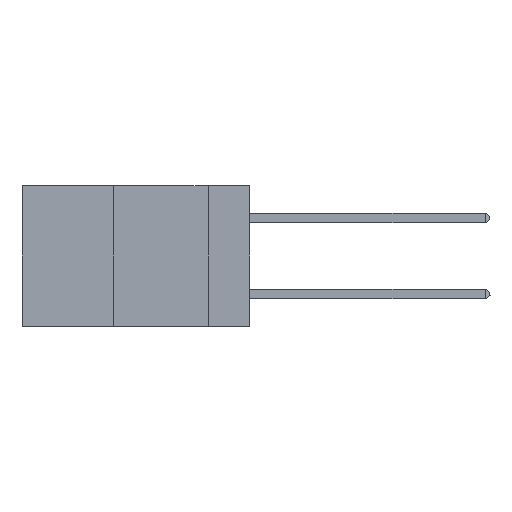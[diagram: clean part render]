
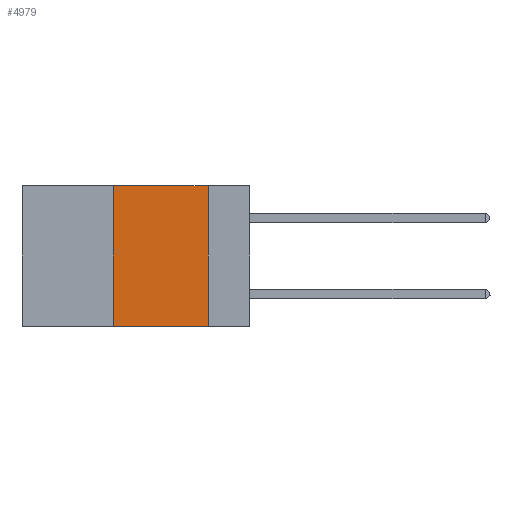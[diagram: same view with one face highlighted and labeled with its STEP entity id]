
A CAD part, left-side view. The second image highlights one B-rep face of the part: STEP entity #4979.
In plain terms, the highlighted planar face has unit normal (-1, 0, 0).
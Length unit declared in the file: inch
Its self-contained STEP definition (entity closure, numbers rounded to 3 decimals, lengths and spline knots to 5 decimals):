
#2656 = LINE ( 'NONE', #20775, #21269 ) ;
#2735 = VERTEX_POINT ( 'NONE', #14490 ) ;
#2810 = VECTOR ( 'NONE', #8553, 39.37008 ) ;
#2898 = CARTESIAN_POINT ( 'NONE',  ( 0., 0.36, 0. ) ) ;
#4979 = ADVANCED_FACE ( 'NONE', ( #11191 ), #26949, .F. ) ;
#6540 = VERTEX_POINT ( 'NONE', #43272 ) ;
#8553 = DIRECTION ( 'NONE',  ( 0., -1., 0. ) ) ;
#8748 = AXIS2_PLACEMENT_3D ( 'NONE', #21558, #14508, #42580 ) ;
#11191 = FACE_OUTER_BOUND ( 'NONE', #39008, .T. ) ;
#11654 = ORIENTED_EDGE ( 'NONE', *, *, #19521, .T. ) ;
#12310 = CARTESIAN_POINT ( 'NONE',  ( 0., 0.36, 0. ) ) ;
#14490 = CARTESIAN_POINT ( 'NONE',  ( 0., 0.36, -0.37 ) ) ;
#14508 = DIRECTION ( 'NONE',  ( 1., 0., 0. ) ) ;
#17548 = VECTOR ( 'NONE', #33337, 39.37008 ) ;
#18623 = VERTEX_POINT ( 'NONE', #24396 ) ;
#19521 = EDGE_CURVE ( 'NONE', #2735, #6540, #2656, .T. ) ;
#20775 = CARTESIAN_POINT ( 'NONE',  ( 0., 0.6, -0.37 ) ) ;
#21269 = VECTOR ( 'NONE', #37691, 39.37008 ) ;
#21558 = CARTESIAN_POINT ( 'NONE',  ( 0., 0.6, 0. ) ) ;
#21889 = VERTEX_POINT ( 'NONE', #12310 ) ;
#23025 = CARTESIAN_POINT ( 'NONE',  ( 0., 0.11, 0. ) ) ;
#23467 = VECTOR ( 'NONE', #35154, 39.37008 ) ;
#24396 = CARTESIAN_POINT ( 'NONE',  ( 0., 0.11, 0. ) ) ;
#25597 = ORIENTED_EDGE ( 'NONE', *, *, #35608, .F. ) ;
#26558 = ORIENTED_EDGE ( 'NONE', *, *, #31101, .F. ) ;
#26857 = LINE ( 'NONE', #23025, #17548 ) ;
#26949 = PLANE ( 'NONE',  #8748 ) ;
#27260 = ORIENTED_EDGE ( 'NONE', *, *, #41774, .F. ) ;
#31101 = EDGE_CURVE ( 'NONE', #2735, #21889, #33593, .T. ) ;
#33337 = DIRECTION ( 'NONE',  ( 0., 0., -1. ) ) ;
#33593 = LINE ( 'NONE', #2898, #23467 ) ;
#35154 = DIRECTION ( 'NONE',  ( 0., 0., 1. ) ) ;
#35608 = EDGE_CURVE ( 'NONE', #18623, #6540, #26857, .T. ) ;
#37691 = DIRECTION ( 'NONE',  ( 0., -1., 0. ) ) ;
#39008 = EDGE_LOOP ( 'NONE', ( #25597, #27260, #26558, #11654 ) ) ;
#39383 = LINE ( 'NONE', #43268, #2810 ) ;
#41774 = EDGE_CURVE ( 'NONE', #21889, #18623, #39383, .T. ) ;
#42580 = DIRECTION ( 'NONE',  ( 0., 0., -1. ) ) ;
#43268 = CARTESIAN_POINT ( 'NONE',  ( 0., 0.6, 0. ) ) ;
#43272 = CARTESIAN_POINT ( 'NONE',  ( 0., 0.11, -0.37 ) ) ;
